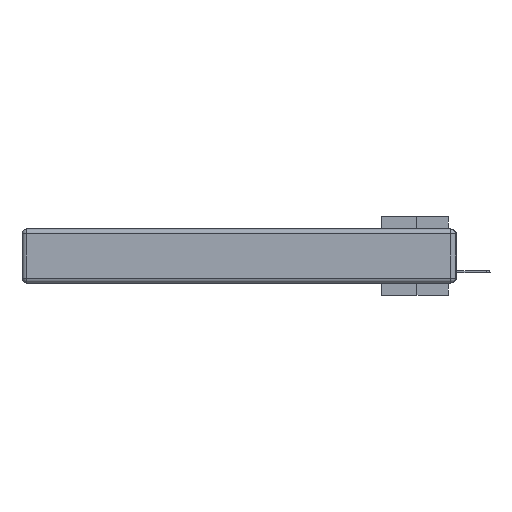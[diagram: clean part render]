
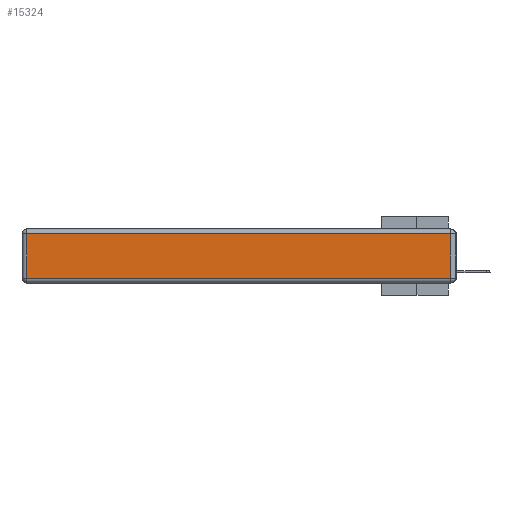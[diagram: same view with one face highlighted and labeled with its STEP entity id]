
A CAD part, left-side view. The second image highlights one B-rep face of the part: STEP entity #15324.
In plain terms, the highlighted planar face has unit normal (-1, 0, 0).
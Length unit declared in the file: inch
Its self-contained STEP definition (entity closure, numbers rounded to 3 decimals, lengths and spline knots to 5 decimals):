
#749 = VECTOR ( 'NONE', #14657, 39.37008 ) ;
#2467 = ORIENTED_EDGE ( 'NONE', *, *, #14866, .T. ) ;
#2728 = LINE ( 'NONE', #20822, #26411 ) ;
#3768 = LINE ( 'NONE', #26854, #18595 ) ;
#4052 = VERTEX_POINT ( 'NONE', #29281 ) ;
#4831 = CARTESIAN_POINT ( 'NONE',  ( 0., 0., -0.343 ) ) ;
#5991 = DIRECTION ( 'NONE',  ( 0., 0., -1. ) ) ;
#7153 = DIRECTION ( 'NONE',  ( 0., 0., 1. ) ) ;
#9101 = EDGE_LOOP ( 'NONE', ( #23939, #2467, #29599, #13438 ) ) ;
#10109 = AXIS2_PLACEMENT_3D ( 'NONE', #4831, #23947, #7153 ) ;
#13438 = ORIENTED_EDGE ( 'NONE', *, *, #21882, .T. ) ;
#14657 = DIRECTION ( 'NONE',  ( 0., 1., 0. ) ) ;
#14866 = EDGE_CURVE ( 'NONE', #15394, #26646, #17619, .T. ) ;
#15324 = ADVANCED_FACE ( 'NONE', ( #30312 ), #18920, .T. ) ;
#15394 = VERTEX_POINT ( 'NONE', #28893 ) ;
#15582 = CARTESIAN_POINT ( 'NONE',  ( 0., 2.72, -0.313 ) ) ;
#17020 = CARTESIAN_POINT ( 'NONE',  ( 0., 2.75, -0.03 ) ) ;
#17619 = LINE ( 'NONE', #23887, #29088 ) ;
#18595 = VECTOR ( 'NONE', #22011, 39.37008 ) ;
#18920 = PLANE ( 'NONE',  #10109 ) ;
#20475 = EDGE_CURVE ( 'NONE', #30172, #15394, #3768, .T. ) ;
#20822 = CARTESIAN_POINT ( 'NONE',  ( 0., 2.72, -0.343 ) ) ;
#21139 = LINE ( 'NONE', #17020, #749 ) ;
#21426 = DIRECTION ( 'NONE',  ( 0., 0., 1. ) ) ;
#21882 = EDGE_CURVE ( 'NONE', #4052, #30172, #2728, .T. ) ;
#22011 = DIRECTION ( 'NONE',  ( 0., -1., 0. ) ) ;
#23393 = EDGE_CURVE ( 'NONE', #26646, #4052, #21139, .T. ) ;
#23887 = CARTESIAN_POINT ( 'NONE',  ( 0., 0.03, -0.343 ) ) ;
#23939 = ORIENTED_EDGE ( 'NONE', *, *, #20475, .T. ) ;
#23947 = DIRECTION ( 'NONE',  ( -1., 0., 0. ) ) ;
#26262 = CARTESIAN_POINT ( 'NONE',  ( 0., 0.03, -0.03 ) ) ;
#26411 = VECTOR ( 'NONE', #5991, 39.37008 ) ;
#26646 = VERTEX_POINT ( 'NONE', #26262 ) ;
#26854 = CARTESIAN_POINT ( 'NONE',  ( 0., 0., -0.313 ) ) ;
#28893 = CARTESIAN_POINT ( 'NONE',  ( 0., 0.03, -0.313 ) ) ;
#29088 = VECTOR ( 'NONE', #21426, 39.37008 ) ;
#29281 = CARTESIAN_POINT ( 'NONE',  ( 0., 2.72, -0.03 ) ) ;
#29599 = ORIENTED_EDGE ( 'NONE', *, *, #23393, .T. ) ;
#30172 = VERTEX_POINT ( 'NONE', #15582 ) ;
#30312 = FACE_OUTER_BOUND ( 'NONE', #9101, .T. ) ;
